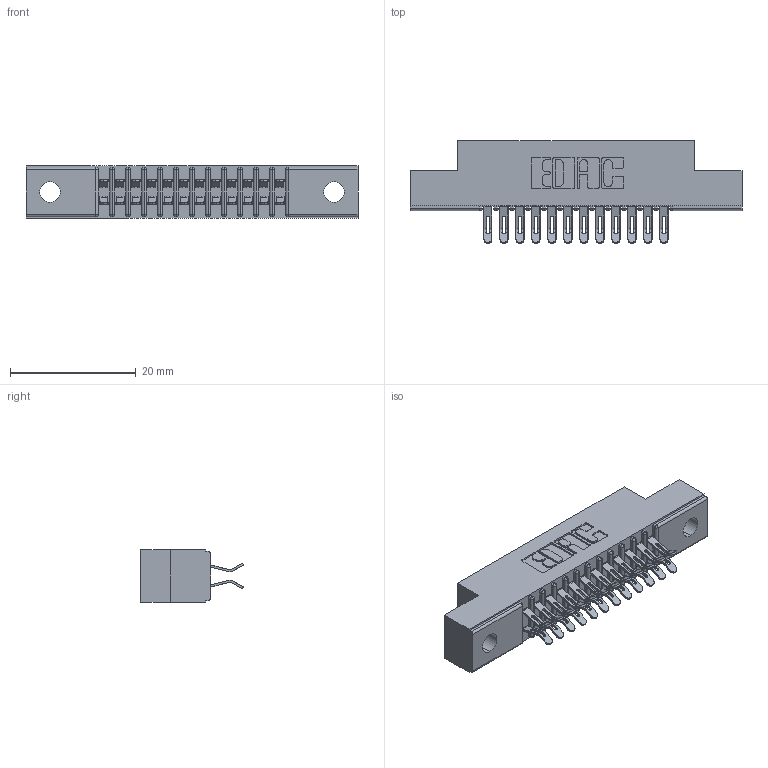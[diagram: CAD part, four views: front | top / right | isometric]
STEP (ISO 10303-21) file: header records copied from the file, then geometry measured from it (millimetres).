
FILE_DESCRIPTION (( 'STEP AP203' ), '1' );
FILE_NAME ('341-024-555-202.STEP', '2018-08-06T18:10:01', ( '' ), ( '' ), 'SwSTEP 2.0', 'SolidWorks 2016', '' );
FILE_SCHEMA (( 'CONFIG_CONTROL_DESIGN' ));
Length unit declared in the file: inch
Products named in the file (3): 341 Part_.128 (3.25) Dia Mounting Holes; 341-292-001_341-292-155; 341-024-555-202
Assembly tree (25 placements, depth 2):
  341-024-555-202
    341 Part_.128 (3.25) Dia Mounting Holes
    341-292-001_341-292-155  x24
Bounding box: 52.7 x 16.31 x 8.38 mm (x, y, z)
Volume: 3018.2 mm3; surface area: 5618.6 mm2
Topology: 25 solids, 25 shells, 1988 faces, 5920 edges, 3854 vertices
Faces by surface type: plane 1076, cylinder 864, sphere 26, torus 22
Entity records: 18991 total; most frequent: CARTESIAN_POINT 3174, ORIENTED_EDGE 3140, DIRECTION 3092, EDGE_CURVE 1570, LINE 1220, VECTOR 1220, VERTEX_POINT 1002, AXIS2_PLACEMENT_3D 936
